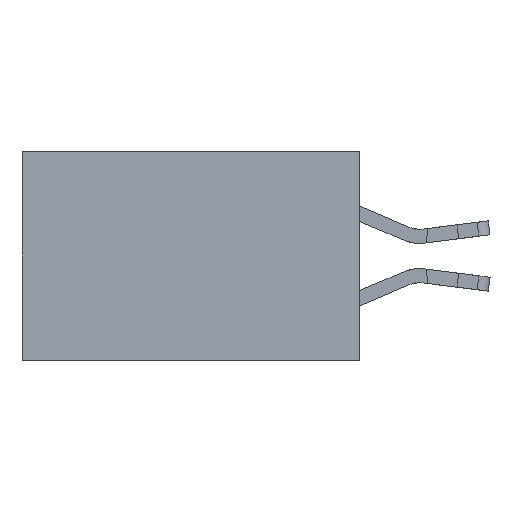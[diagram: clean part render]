
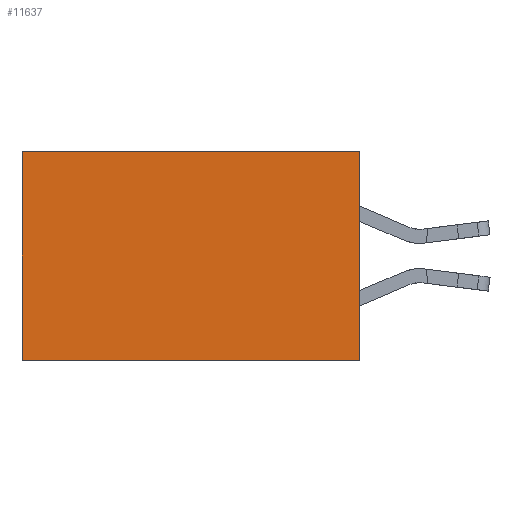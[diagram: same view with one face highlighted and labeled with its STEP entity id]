
A CAD part, left-side view. The second image highlights one B-rep face of the part: STEP entity #11637.
In plain terms, the highlighted planar face has unit normal (-1, 0, 0).
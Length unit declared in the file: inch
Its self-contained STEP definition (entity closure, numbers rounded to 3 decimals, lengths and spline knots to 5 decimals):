
#1264 = VERTEX_POINT ( 'NONE', #14010 ) ;
#1349 = ORIENTED_EDGE ( 'NONE', *, *, #9770, .F. ) ;
#1511 = VERTEX_POINT ( 'NONE', #2165 ) ;
#2165 = CARTESIAN_POINT ( 'NONE',  ( 0.2875, 0.6, 0. ) ) ;
#2454 = EDGE_LOOP ( 'NONE', ( #4532, #1349, #6659, #3540 ) ) ;
#3436 = VECTOR ( 'NONE', #6947, 39.37008 ) ;
#3540 = ORIENTED_EDGE ( 'NONE', *, *, #3591, .T. ) ;
#3591 = EDGE_CURVE ( 'NONE', #14007, #1511, #5075, .T. ) ;
#4119 = CARTESIAN_POINT ( 'NONE',  ( 0.2875, 0., 0. ) ) ;
#4532 = ORIENTED_EDGE ( 'NONE', *, *, #9114, .T. ) ;
#5075 = LINE ( 'NONE', #4119, #3436 ) ;
#5242 = PLANE ( 'NONE',  #7716 ) ;
#5477 = DIRECTION ( 'NONE',  ( 0., 1., 0. ) ) ;
#5775 = CARTESIAN_POINT ( 'NONE',  ( 0.2875, 0.6, 0. ) ) ;
#6659 = ORIENTED_EDGE ( 'NONE', *, *, #7076, .F. ) ;
#6850 = CARTESIAN_POINT ( 'NONE',  ( 0.2875, 0., -0.37 ) ) ;
#6947 = DIRECTION ( 'NONE',  ( 0., 1., 0. ) ) ;
#7076 = EDGE_CURVE ( 'NONE', #14007, #1264, #11014, .T. ) ;
#7716 = AXIS2_PLACEMENT_3D ( 'NONE', #15720, #9610, #11115 ) ;
#9114 = EDGE_CURVE ( 'NONE', #1511, #18628, #17212, .T. ) ;
#9310 = VECTOR ( 'NONE', #16793, 39.37008 ) ;
#9610 = DIRECTION ( 'NONE',  ( 1., 0., 0. ) ) ;
#9770 = EDGE_CURVE ( 'NONE', #1264, #18628, #15333, .T. ) ;
#11014 = LINE ( 'NONE', #13595, #17731 ) ;
#11115 = DIRECTION ( 'NONE',  ( 0., 0., -1. ) ) ;
#11637 = ADVANCED_FACE ( 'NONE', ( #18024 ), #5242, .F. ) ;
#12286 = DIRECTION ( 'NONE',  ( 0., 0., -1. ) ) ;
#12359 = CARTESIAN_POINT ( 'NONE',  ( 0.2875, 0.6, -0.37 ) ) ;
#12479 = CARTESIAN_POINT ( 'NONE',  ( 0.2875, 0., 0. ) ) ;
#13595 = CARTESIAN_POINT ( 'NONE',  ( 0.2875, 0., 0. ) ) ;
#14007 = VERTEX_POINT ( 'NONE', #12479 ) ;
#14010 = CARTESIAN_POINT ( 'NONE',  ( 0.2875, 0., -0.37 ) ) ;
#15108 = VECTOR ( 'NONE', #5477, 39.37008 ) ;
#15333 = LINE ( 'NONE', #6850, #15108 ) ;
#15720 = CARTESIAN_POINT ( 'NONE',  ( 0.2875, 0., 0. ) ) ;
#16793 = DIRECTION ( 'NONE',  ( 0., 0., -1. ) ) ;
#17212 = LINE ( 'NONE', #5775, #9310 ) ;
#17731 = VECTOR ( 'NONE', #12286, 39.37008 ) ;
#18024 = FACE_OUTER_BOUND ( 'NONE', #2454, .T. ) ;
#18628 = VERTEX_POINT ( 'NONE', #12359 ) ;
